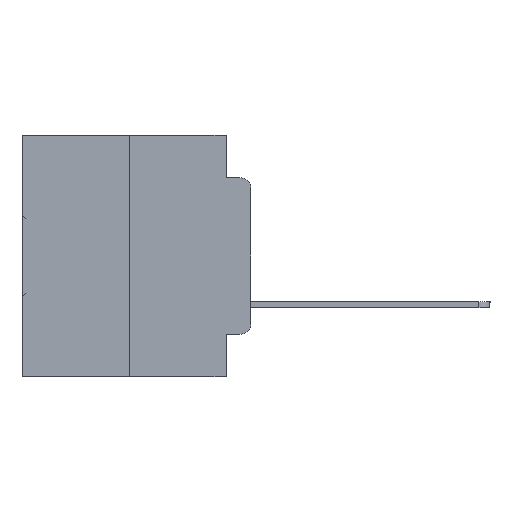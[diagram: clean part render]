
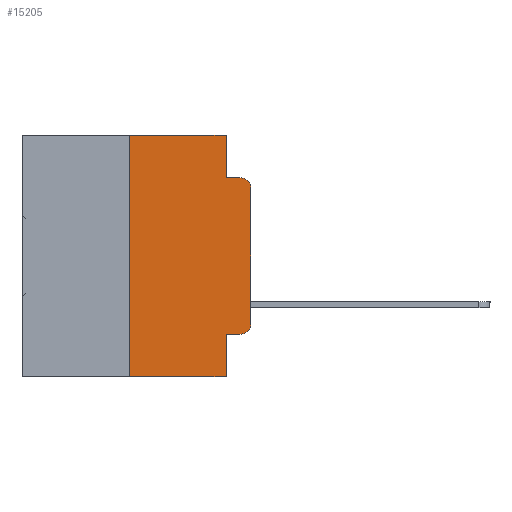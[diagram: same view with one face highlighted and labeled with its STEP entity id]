
A CAD part, left-side view. The second image highlights one B-rep face of the part: STEP entity #15205.
In plain terms, the highlighted planar face has unit normal (-1, 0, 0).
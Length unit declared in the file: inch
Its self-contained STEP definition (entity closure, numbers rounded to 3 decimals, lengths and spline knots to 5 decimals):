
#555 = LINE ( 'NONE', #10608, #17038 ) ;
#1030 = EDGE_CURVE ( 'NONE', #9739, #12918, #1651, .T. ) ;
#1138 = EDGE_LOOP ( 'NONE', ( #1636, #26156, #17557, #21010, #18722, #30714, #21979, #13944, #29597, #12517 ) ) ;
#1423 = DIRECTION ( 'NONE',  ( 0., -1., 0. ) ) ;
#1452 = CARTESIAN_POINT ( 'NONE',  ( 0., 0.25, 0. ) ) ;
#1534 = CARTESIAN_POINT ( 'NONE',  ( 0., 0.051, -0.0885 ) ) ;
#1636 = ORIENTED_EDGE ( 'NONE', *, *, #25359, .T. ) ;
#1651 = CIRCLE ( 'NONE', #20756, 0.02 ) ;
#1955 = VERTEX_POINT ( 'NONE', #13437 ) ;
#2735 = LINE ( 'NONE', #10577, #18432 ) ;
#3535 = EDGE_CURVE ( 'NONE', #17206, #12918, #12799, .T. ) ;
#3568 = VECTOR ( 'NONE', #12585, 39.37008 ) ;
#4998 = CARTESIAN_POINT ( 'NONE',  ( 0., 0., -0.1085 ) ) ;
#5465 = DIRECTION ( 'NONE',  ( 0., 0., 1. ) ) ;
#6252 = DIRECTION ( 'NONE',  ( 0., 0., -1. ) ) ;
#6704 = CARTESIAN_POINT ( 'NONE',  ( 0., 0.02, -0.1085 ) ) ;
#7469 = CARTESIAN_POINT ( 'NONE',  ( 0., 0.473, 0. ) ) ;
#8187 = DIRECTION ( 'NONE',  ( 0., -1., 0. ) ) ;
#8234 = VECTOR ( 'NONE', #12687, 39.37008 ) ;
#8250 = CARTESIAN_POINT ( 'NONE',  ( 0., 0., 0. ) ) ;
#8738 = VECTOR ( 'NONE', #30266, 39.37008 ) ;
#9306 = AXIS2_PLACEMENT_3D ( 'NONE', #11864, #22323, #6252 ) ;
#9520 = CARTESIAN_POINT ( 'NONE',  ( 0., 0.051, 0. ) ) ;
#9739 = VERTEX_POINT ( 'NONE', #4998 ) ;
#9934 = EDGE_CURVE ( 'NONE', #22364, #26582, #555, .T. ) ;
#9958 = LINE ( 'NONE', #22965, #8234 ) ;
#10559 = CARTESIAN_POINT ( 'NONE',  ( 0., 0.25, -0.5 ) ) ;
#10577 = CARTESIAN_POINT ( 'NONE',  ( 0., 0.25, 0. ) ) ;
#10596 = CARTESIAN_POINT ( 'NONE',  ( 0., 0., -0.3915 ) ) ;
#10608 = CARTESIAN_POINT ( 'NONE',  ( 0., 0.051, -0.4115 ) ) ;
#11616 = EDGE_CURVE ( 'NONE', #30311, #13517, #30316, .T. ) ;
#11864 = CARTESIAN_POINT ( 'NONE',  ( 0., 0.02, -0.3915 ) ) ;
#12080 = PLANE ( 'NONE',  #21556 ) ;
#12415 = DIRECTION ( 'NONE',  ( 1., 0., 0. ) ) ;
#12517 = ORIENTED_EDGE ( 'NONE', *, *, #32841, .T. ) ;
#12585 = DIRECTION ( 'NONE',  ( 0., 0., -1. ) ) ;
#12687 = DIRECTION ( 'NONE',  ( 0., 0., -1. ) ) ;
#12799 = LINE ( 'NONE', #15552, #28303 ) ;
#12918 = VERTEX_POINT ( 'NONE', #25186 ) ;
#13291 = CARTESIAN_POINT ( 'NONE',  ( 0., 0.02, -0.4115 ) ) ;
#13437 = CARTESIAN_POINT ( 'NONE',  ( 0., 0.051, 0. ) ) ;
#13517 = VERTEX_POINT ( 'NONE', #30861 ) ;
#13944 = ORIENTED_EDGE ( 'NONE', *, *, #15183, .F. ) ;
#14074 = DIRECTION ( 'NONE',  ( 0., 0., -1. ) ) ;
#15183 = EDGE_CURVE ( 'NONE', #22364, #13517, #33307, .T. ) ;
#15205 = ADVANCED_FACE ( 'NONE', ( #28348 ), #12080, .F. ) ;
#15311 = CIRCLE ( 'NONE', #9306, 0.02 ) ;
#15552 = CARTESIAN_POINT ( 'NONE',  ( 0., 0.051, -0.0885 ) ) ;
#16048 = VECTOR ( 'NONE', #1423, 39.37008 ) ;
#17038 = VECTOR ( 'NONE', #23461, 39.37008 ) ;
#17206 = VERTEX_POINT ( 'NONE', #1534 ) ;
#17557 = ORIENTED_EDGE ( 'NONE', *, *, #3535, .F. ) ;
#17981 = VERTEX_POINT ( 'NONE', #1452 ) ;
#18432 = VECTOR ( 'NONE', #5465, 39.37008 ) ;
#18722 = ORIENTED_EDGE ( 'NONE', *, *, #31893, .F. ) ;
#19670 = LINE ( 'NONE', #32331, #8738 ) ;
#20096 = VECTOR ( 'NONE', #28961, 39.37008 ) ;
#20756 = AXIS2_PLACEMENT_3D ( 'NONE', #6704, #32705, #14074 ) ;
#21010 = ORIENTED_EDGE ( 'NONE', *, *, #29636, .F. ) ;
#21247 = VERTEX_POINT ( 'NONE', #10596 ) ;
#21556 = AXIS2_PLACEMENT_3D ( 'NONE', #7469, #12415, #27212 ) ;
#21979 = ORIENTED_EDGE ( 'NONE', *, *, #11616, .T. ) ;
#22323 = DIRECTION ( 'NONE',  ( -1., 0., 0. ) ) ;
#22364 = VERTEX_POINT ( 'NONE', #22383 ) ;
#22383 = CARTESIAN_POINT ( 'NONE',  ( 0., 0.051, -0.4115 ) ) ;
#22965 = CARTESIAN_POINT ( 'NONE',  ( 0., 0.051, 0. ) ) ;
#23461 = DIRECTION ( 'NONE',  ( 0., -1., 0. ) ) ;
#23650 = LINE ( 'NONE', #8250, #20096 ) ;
#25186 = CARTESIAN_POINT ( 'NONE',  ( 0., 0.02, -0.0885 ) ) ;
#25359 = EDGE_CURVE ( 'NONE', #21247, #9739, #23650, .T. ) ;
#25997 = EDGE_CURVE ( 'NONE', #30311, #17981, #2735, .T. ) ;
#26156 = ORIENTED_EDGE ( 'NONE', *, *, #1030, .T. ) ;
#26582 = VERTEX_POINT ( 'NONE', #13291 ) ;
#27212 = DIRECTION ( 'NONE',  ( 0., 0., -1. ) ) ;
#28303 = VECTOR ( 'NONE', #8187, 39.37008 ) ;
#28348 = FACE_OUTER_BOUND ( 'NONE', #1138, .T. ) ;
#28961 = DIRECTION ( 'NONE',  ( 0., 0., 1. ) ) ;
#29597 = ORIENTED_EDGE ( 'NONE', *, *, #9934, .T. ) ;
#29636 = EDGE_CURVE ( 'NONE', #1955, #17206, #9958, .T. ) ;
#29989 = CARTESIAN_POINT ( 'NONE',  ( 0., 0.473, -0.5 ) ) ;
#30266 = DIRECTION ( 'NONE',  ( 0., -1., 0. ) ) ;
#30311 = VERTEX_POINT ( 'NONE', #10559 ) ;
#30316 = LINE ( 'NONE', #29989, #16048 ) ;
#30714 = ORIENTED_EDGE ( 'NONE', *, *, #25997, .F. ) ;
#30861 = CARTESIAN_POINT ( 'NONE',  ( 0., 0.051, -0.5 ) ) ;
#31893 = EDGE_CURVE ( 'NONE', #17981, #1955, #19670, .T. ) ;
#32331 = CARTESIAN_POINT ( 'NONE',  ( 0., 0.473, 0. ) ) ;
#32705 = DIRECTION ( 'NONE',  ( -1., 0., 0. ) ) ;
#32841 = EDGE_CURVE ( 'NONE', #26582, #21247, #15311, .T. ) ;
#33307 = LINE ( 'NONE', #9520, #3568 ) ;
